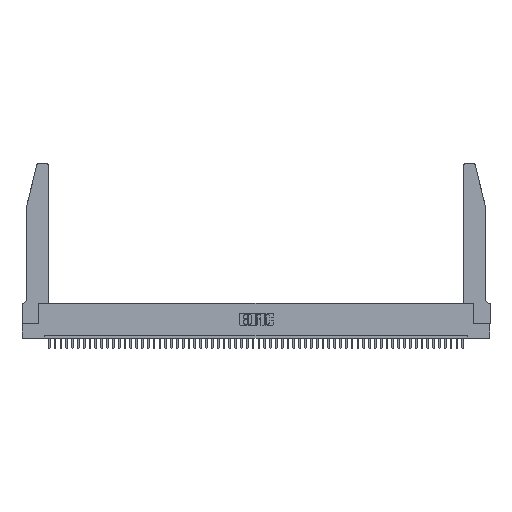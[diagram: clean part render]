
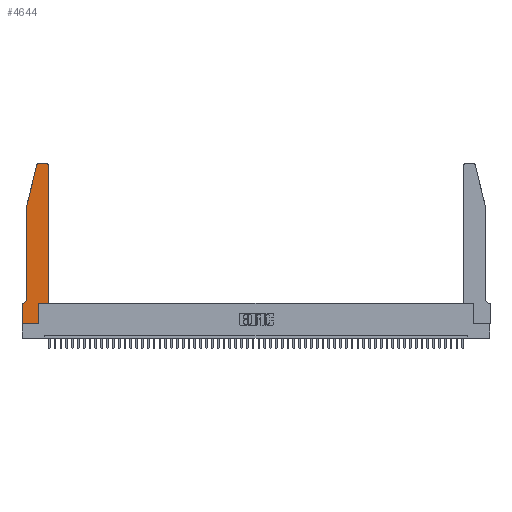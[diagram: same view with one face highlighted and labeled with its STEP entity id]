
A CAD part, top view. The second image highlights one B-rep face of the part: STEP entity #4644.
In plain terms, the highlighted planar face has unit normal (0, 0, 1).
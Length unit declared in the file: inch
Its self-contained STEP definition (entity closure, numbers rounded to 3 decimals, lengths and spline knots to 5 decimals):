
#385 = ORIENTED_EDGE ( 'NONE', *, *, #33495, .T. ) ;
#737 = DIRECTION ( 'NONE',  ( 1., 0., 0. ) ) ;
#1872 = VERTEX_POINT ( 'NONE', #6628 ) ;
#2242 = DIRECTION ( 'NONE',  ( 1., 0., 0. ) ) ;
#2440 = AXIS2_PLACEMENT_3D ( 'NONE', #21037, #29166, #12499 ) ;
#2896 = EDGE_CURVE ( 'NONE', #34647, #20356, #49390, .T. ) ;
#3606 = CARTESIAN_POINT ( 'NONE',  ( 0., 0., 0.37 ) ) ;
#3770 = DIRECTION ( 'NONE',  ( 0., -1., 0. ) ) ;
#4398 = CIRCLE ( 'NONE', #35264, 0.03 ) ;
#4644 = ADVANCED_FACE ( 'NONE', ( #15284 ), #20657, .T. ) ;
#4738 = CARTESIAN_POINT ( 'NONE',  ( 0.2865, 0.35, 0.37 ) ) ;
#5303 = VERTEX_POINT ( 'NONE', #14800 ) ;
#5987 = DIRECTION ( 'NONE',  ( 0., 0., 1. ) ) ;
#6545 = CARTESIAN_POINT ( 'NONE',  ( 0.284, 2.72, 0.37 ) ) ;
#6628 = CARTESIAN_POINT ( 'NONE',  ( 0.4505, 0.35, 0.37 ) ) ;
#6790 = CARTESIAN_POINT ( 'NONE',  ( 0.2865, 0.35, 0.37 ) ) ;
#7627 = EDGE_CURVE ( 'NONE', #10347, #30962, #17660, .T. ) ;
#7798 = EDGE_CURVE ( 'NONE', #1872, #10347, #46851, .T. ) ;
#7967 = DIRECTION ( 'NONE',  ( -0.239, -0.971, 0. ) ) ;
#8231 = VERTEX_POINT ( 'NONE', #36868 ) ;
#8375 = ORIENTED_EDGE ( 'NONE', *, *, #10492, .T. ) ;
#8500 = EDGE_LOOP ( 'NONE', ( #11754, #30383, #35870, #52042, #8375, #9984, #43949, #385, #36592, #14224, #43507, #20231 ) ) ;
#8504 = DIRECTION ( 'NONE',  ( 1., 0., 0. ) ) ;
#9914 = VECTOR ( 'NONE', #51063, 39.37008 ) ;
#9984 = ORIENTED_EDGE ( 'NONE', *, *, #13509, .T. ) ;
#10347 = VERTEX_POINT ( 'NONE', #48086 ) ;
#10492 = EDGE_CURVE ( 'NONE', #20356, #8231, #52017, .T. ) ;
#11754 = ORIENTED_EDGE ( 'NONE', *, *, #12676, .T. ) ;
#12499 = DIRECTION ( 'NONE',  ( 1., 0., 0. ) ) ;
#12676 = EDGE_CURVE ( 'NONE', #30962, #5303, #48401, .T. ) ;
#12691 = LINE ( 'NONE', #6790, #30605 ) ;
#12875 = VERTEX_POINT ( 'NONE', #13883 ) ;
#13509 = EDGE_CURVE ( 'NONE', #8231, #41116, #46335, .T. ) ;
#13883 = CARTESIAN_POINT ( 'NONE',  ( 0., 0., 0.37 ) ) ;
#13984 = EDGE_CURVE ( 'NONE', #41116, #12875, #38940, .T. ) ;
#14224 = ORIENTED_EDGE ( 'NONE', *, *, #22497, .T. ) ;
#14559 = LINE ( 'NONE', #24448, #47119 ) ;
#14800 = CARTESIAN_POINT ( 'NONE',  ( 0.284, 2.75, 0.37 ) ) ;
#15276 = VERTEX_POINT ( 'NONE', #4738 ) ;
#15284 = FACE_OUTER_BOUND ( 'NONE', #8500, .T. ) ;
#15576 = CARTESIAN_POINT ( 'NONE',  ( 0.0755, 2., 0.37 ) ) ;
#15766 = CARTESIAN_POINT ( 'NONE',  ( 0.0055, 0.42, 0.37 ) ) ;
#15945 = DIRECTION ( 'NONE',  ( -1., 0., 0. ) ) ;
#16230 = DIRECTION ( 'NONE',  ( 1., 0., 0. ) ) ;
#16734 = VECTOR ( 'NONE', #737, 39.37008 ) ;
#17660 = CIRCLE ( 'NONE', #45930, 0.03 ) ;
#19698 = EDGE_CURVE ( 'NONE', #5303, #24776, #4398, .T. ) ;
#19702 = VECTOR ( 'NONE', #3770, 39.37008 ) ;
#20231 = ORIENTED_EDGE ( 'NONE', *, *, #7627, .T. ) ;
#20356 = VERTEX_POINT ( 'NONE', #50864 ) ;
#20509 = CARTESIAN_POINT ( 'NONE',  ( 0.2865, 0., 0.37 ) ) ;
#20657 = PLANE ( 'NONE',  #2440 ) ;
#21037 = CARTESIAN_POINT ( 'NONE',  ( 0., 0.35, 0.37 ) ) ;
#21968 = CARTESIAN_POINT ( 'NONE',  ( 0.0755, 0.35, 0.37 ) ) ;
#22497 = EDGE_CURVE ( 'NONE', #15276, #1872, #47237, .T. ) ;
#22896 = CARTESIAN_POINT ( 'NONE',  ( 0.4505, 0.35, 0.37 ) ) ;
#24448 = CARTESIAN_POINT ( 'NONE',  ( 0.0755, 2., 0.37 ) ) ;
#24776 = VERTEX_POINT ( 'NONE', #43560 ) ;
#24917 = VERTEX_POINT ( 'NONE', #20509 ) ;
#25075 = CARTESIAN_POINT ( 'NONE',  ( 0., 0., 0.37 ) ) ;
#25209 = CARTESIAN_POINT ( 'NONE',  ( 0.2605, 2.75, 0.37 ) ) ;
#27847 = AXIS2_PLACEMENT_3D ( 'NONE', #15766, #49563, #15945 ) ;
#28222 = VECTOR ( 'NONE', #43909, 39.37008 ) ;
#29166 = DIRECTION ( 'NONE',  ( 0., 0., 1. ) ) ;
#30383 = ORIENTED_EDGE ( 'NONE', *, *, #19698, .T. ) ;
#30605 = VECTOR ( 'NONE', #32727, 39.37008 ) ;
#30962 = VERTEX_POINT ( 'NONE', #47648 ) ;
#32727 = DIRECTION ( 'NONE',  ( 0., 1., 0. ) ) ;
#33495 = EDGE_CURVE ( 'NONE', #12875, #24917, #41297, .T. ) ;
#34647 = VERTEX_POINT ( 'NONE', #15576 ) ;
#35264 = AXIS2_PLACEMENT_3D ( 'NONE', #6545, #5987, #2242 ) ;
#35870 = ORIENTED_EDGE ( 'NONE', *, *, #51148, .T. ) ;
#36592 = ORIENTED_EDGE ( 'NONE', *, *, #50113, .T. ) ;
#36868 = CARTESIAN_POINT ( 'NONE',  ( 0.0055, 0.35, 0.37 ) ) ;
#37427 = CARTESIAN_POINT ( 'NONE',  ( 0.4205, 2.72, 0.37 ) ) ;
#38940 = LINE ( 'NONE', #25075, #19702 ) ;
#41116 = VERTEX_POINT ( 'NONE', #54723 ) ;
#41297 = LINE ( 'NONE', #3606, #48587 ) ;
#43507 = ORIENTED_EDGE ( 'NONE', *, *, #7798, .T. ) ;
#43560 = CARTESIAN_POINT ( 'NONE',  ( 0.25487, 2.72718, 0.37 ) ) ;
#43909 = DIRECTION ( 'NONE',  ( 0., 1., 0. ) ) ;
#43949 = ORIENTED_EDGE ( 'NONE', *, *, #13984, .T. ) ;
#44321 = DIRECTION ( 'NONE',  ( 0., -1., 0. ) ) ;
#45930 = AXIS2_PLACEMENT_3D ( 'NONE', #37427, #50650, #8504 ) ;
#46335 = LINE ( 'NONE', #21968, #47671 ) ;
#46716 = VECTOR ( 'NONE', #44321, 39.37008 ) ;
#46851 = LINE ( 'NONE', #22896, #28222 ) ;
#47119 = VECTOR ( 'NONE', #7967, 39.37008 ) ;
#47237 = LINE ( 'NONE', #47896, #16734 ) ;
#47648 = CARTESIAN_POINT ( 'NONE',  ( 0.4205, 2.75, 0.37 ) ) ;
#47671 = VECTOR ( 'NONE', #51683, 39.37008 ) ;
#47896 = CARTESIAN_POINT ( 'NONE',  ( 0.4505, 0.35, 0.37 ) ) ;
#48086 = CARTESIAN_POINT ( 'NONE',  ( 0.4505, 2.72, 0.37 ) ) ;
#48401 = LINE ( 'NONE', #25209, #9914 ) ;
#48587 = VECTOR ( 'NONE', #16230, 39.37008 ) ;
#48759 = CARTESIAN_POINT ( 'NONE',  ( 0.0755, 2., 0.37 ) ) ;
#49390 = LINE ( 'NONE', #48759, #46716 ) ;
#49563 = DIRECTION ( 'NONE',  ( 0., 0., -1. ) ) ;
#50113 = EDGE_CURVE ( 'NONE', #24917, #15276, #12691, .T. ) ;
#50650 = DIRECTION ( 'NONE',  ( 0., 0., 1. ) ) ;
#50864 = CARTESIAN_POINT ( 'NONE',  ( 0.0755, 0.42, 0.37 ) ) ;
#51063 = DIRECTION ( 'NONE',  ( -1., 0., 0. ) ) ;
#51148 = EDGE_CURVE ( 'NONE', #24776, #34647, #14559, .T. ) ;
#51683 = DIRECTION ( 'NONE',  ( -1., 0., 0. ) ) ;
#52017 = CIRCLE ( 'NONE', #27847, 0.07 ) ;
#52042 = ORIENTED_EDGE ( 'NONE', *, *, #2896, .T. ) ;
#54723 = CARTESIAN_POINT ( 'NONE',  ( 0., 0.35, 0.37 ) ) ;
